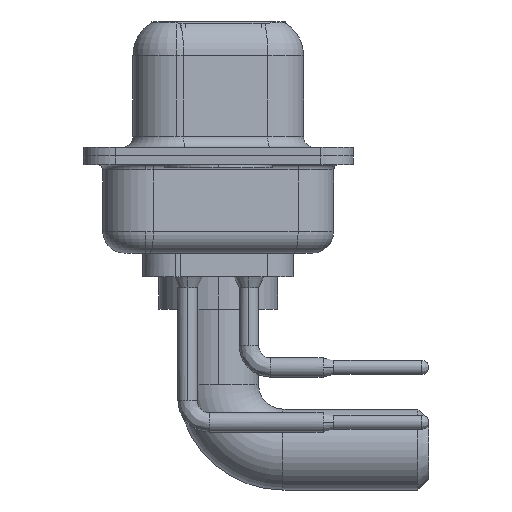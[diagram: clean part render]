
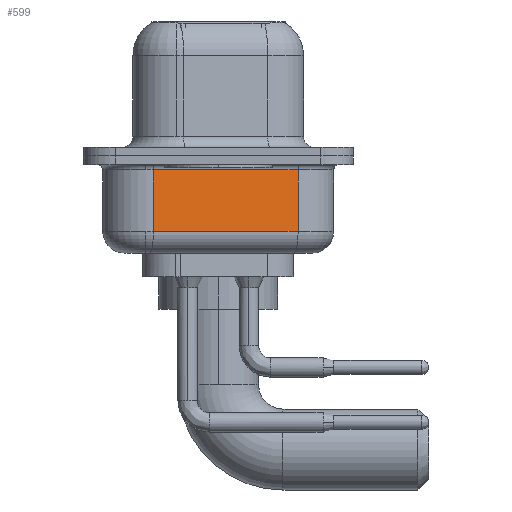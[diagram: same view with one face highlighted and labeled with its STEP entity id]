
A CAD part, left-side view. The second image highlights one B-rep face of the part: STEP entity #599.
In plain terms, the highlighted planar face has unit normal (-0.985, -0.174, 0).
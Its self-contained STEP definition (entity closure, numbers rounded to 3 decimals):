
#281 = LINE ( 'NONE', #9176, #12602 ) ;
#599 = ADVANCED_FACE ( 'NONE', ( #15588 ), #11877, .F. ) ;
#811 = LINE ( 'NONE', #9719, #4294 ) ;
#932 = VECTOR ( 'NONE', #14995, 1000. ) ;
#976 = DIRECTION ( 'NONE',  ( 0.174, -0.985, 0. ) ) ;
#1112 = ORIENTED_EDGE ( 'NONE', *, *, #12062, .T. ) ;
#1634 = EDGE_CURVE ( 'NONE', #5542, #10403, #1964, .T. ) ;
#1964 = LINE ( 'NONE', #12392, #932 ) ;
#2211 = CARTESIAN_POINT ( 'NONE',  ( 4.062, -3.697, -3.5 ) ) ;
#2729 = AXIS2_PLACEMENT_3D ( 'NONE', #6726, #2960, #14240 ) ;
#2960 = DIRECTION ( 'NONE',  ( 0.985, 0.174, 0. ) ) ;
#4294 = VECTOR ( 'NONE', #976, 1000. ) ;
#4513 = CARTESIAN_POINT ( 'NONE',  ( 4.062, -3.697, -0.65 ) ) ;
#5542 = VERTEX_POINT ( 'NONE', #2211 ) ;
#6025 = VERTEX_POINT ( 'NONE', #8643 ) ;
#6441 = CARTESIAN_POINT ( 'NONE',  ( 2.88, 3.003, -3.5 ) ) ;
#6726 = CARTESIAN_POINT ( 'NONE',  ( 2.88, 3.003, -4.5 ) ) ;
#6737 = DIRECTION ( 'NONE',  ( 0., 0., 1. ) ) ;
#7705 = ORIENTED_EDGE ( 'NONE', *, *, #1634, .T. ) ;
#8176 = EDGE_CURVE ( 'NONE', #10403, #6025, #15673, .T. ) ;
#8643 = CARTESIAN_POINT ( 'NONE',  ( 2.88, 3.003, -0.65 ) ) ;
#9023 = VERTEX_POINT ( 'NONE', #6441 ) ;
#9176 = CARTESIAN_POINT ( 'NONE',  ( 2.88, 3.003, -4.5 ) ) ;
#9719 = CARTESIAN_POINT ( 'NONE',  ( 2.88, 3.003, -3.5 ) ) ;
#10403 = VERTEX_POINT ( 'NONE', #4513 ) ;
#11219 = EDGE_CURVE ( 'NONE', #9023, #6025, #281, .T. ) ;
#11877 = PLANE ( 'NONE',  #2729 ) ;
#12062 = EDGE_CURVE ( 'NONE', #9023, #5542, #811, .T. ) ;
#12064 = ORIENTED_EDGE ( 'NONE', *, *, #11219, .F. ) ;
#12129 = EDGE_LOOP ( 'NONE', ( #12064, #1112, #7705, #12267 ) ) ;
#12267 = ORIENTED_EDGE ( 'NONE', *, *, #8176, .T. ) ;
#12392 = CARTESIAN_POINT ( 'NONE',  ( 4.062, -3.697, -4.5 ) ) ;
#12602 = VECTOR ( 'NONE', #6737, 1000. ) ;
#12897 = CARTESIAN_POINT ( 'NONE',  ( 2.88, 3.003, -0.65 ) ) ;
#13598 = VECTOR ( 'NONE', #14159, 1000. ) ;
#14159 = DIRECTION ( 'NONE',  ( -0.174, 0.985, 0. ) ) ;
#14240 = DIRECTION ( 'NONE',  ( -0.174, 0.985, 0. ) ) ;
#14995 = DIRECTION ( 'NONE',  ( 0., 0., 1. ) ) ;
#15588 = FACE_OUTER_BOUND ( 'NONE', #12129, .T. ) ;
#15673 = LINE ( 'NONE', #12897, #13598 ) ;
